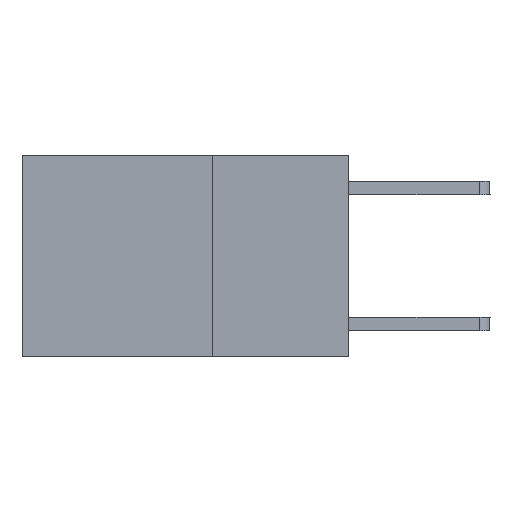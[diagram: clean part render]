
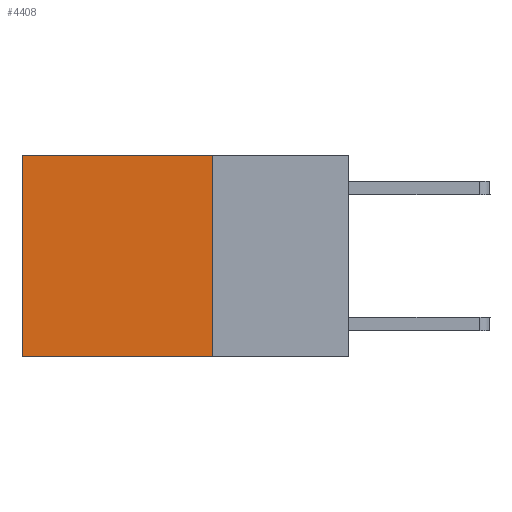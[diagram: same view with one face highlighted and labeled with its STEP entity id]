
A CAD part, left-side view. The second image highlights one B-rep face of the part: STEP entity #4408.
In plain terms, the highlighted planar face has unit normal (-1, 0, 0).
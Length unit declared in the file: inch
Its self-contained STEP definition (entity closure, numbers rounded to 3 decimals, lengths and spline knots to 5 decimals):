
#588 = DIRECTION ( 'NONE',  ( 0., 0., -1. ) ) ;
#1157 = CARTESIAN_POINT ( 'NONE',  ( 0.2625, 0.25, 0. ) ) ;
#1359 = VECTOR ( 'NONE', #5323, 39.37008 ) ;
#1905 = DIRECTION ( 'NONE',  ( 0., 1., 0. ) ) ;
#2230 = CARTESIAN_POINT ( 'NONE',  ( 0.2625, 0.25, -0.37 ) ) ;
#2257 = EDGE_CURVE ( 'NONE', #3905, #7599, #3227, .T. ) ;
#2892 = LINE ( 'NONE', #8716, #9701 ) ;
#3227 = LINE ( 'NONE', #8413, #5267 ) ;
#3594 = CARTESIAN_POINT ( 'NONE',  ( 0.2625, 0.6, 0. ) ) ;
#3823 = LINE ( 'NONE', #6986, #8851 ) ;
#3905 = VERTEX_POINT ( 'NONE', #2230 ) ;
#4408 = ADVANCED_FACE ( 'NONE', ( #7164 ), #6533, .F. ) ;
#4663 = ORIENTED_EDGE ( 'NONE', *, *, #2257, .F. ) ;
#4764 = ORIENTED_EDGE ( 'NONE', *, *, #5033, .T. ) ;
#5033 = EDGE_CURVE ( 'NONE', #5371, #9205, #2892, .T. ) ;
#5267 = VECTOR ( 'NONE', #1905, 39.37008 ) ;
#5323 = DIRECTION ( 'NONE',  ( 0., 0., -1. ) ) ;
#5371 = VERTEX_POINT ( 'NONE', #9681 ) ;
#5460 = DIRECTION ( 'NONE',  ( 0., 0., -1. ) ) ;
#5499 = EDGE_LOOP ( 'NONE', ( #8890, #4663, #9082, #4764 ) ) ;
#5514 = CARTESIAN_POINT ( 'NONE',  ( 0.2625, 0.25, 0. ) ) ;
#6533 = PLANE ( 'NONE',  #9937 ) ;
#6721 = EDGE_CURVE ( 'NONE', #5371, #3905, #10315, .T. ) ;
#6986 = CARTESIAN_POINT ( 'NONE',  ( 0.2625, 0.6, 0. ) ) ;
#7067 = DIRECTION ( 'NONE',  ( 0., 1., 0. ) ) ;
#7164 = FACE_OUTER_BOUND ( 'NONE', #5499, .T. ) ;
#7314 = CARTESIAN_POINT ( 'NONE',  ( 0.2625, 0.6, -0.37 ) ) ;
#7599 = VERTEX_POINT ( 'NONE', #7314 ) ;
#8413 = CARTESIAN_POINT ( 'NONE',  ( 0.2625, 0.25, -0.37 ) ) ;
#8716 = CARTESIAN_POINT ( 'NONE',  ( 0.2625, 0.25, 0. ) ) ;
#8851 = VECTOR ( 'NONE', #588, 39.37008 ) ;
#8890 = ORIENTED_EDGE ( 'NONE', *, *, #9348, .T. ) ;
#9082 = ORIENTED_EDGE ( 'NONE', *, *, #6721, .F. ) ;
#9205 = VERTEX_POINT ( 'NONE', #3594 ) ;
#9348 = EDGE_CURVE ( 'NONE', #9205, #7599, #3823, .T. ) ;
#9681 = CARTESIAN_POINT ( 'NONE',  ( 0.2625, 0.25, 0. ) ) ;
#9701 = VECTOR ( 'NONE', #7067, 39.37008 ) ;
#9937 = AXIS2_PLACEMENT_3D ( 'NONE', #5514, #10385, #5460 ) ;
#10315 = LINE ( 'NONE', #1157, #1359 ) ;
#10385 = DIRECTION ( 'NONE',  ( 1., 0., 0. ) ) ;
